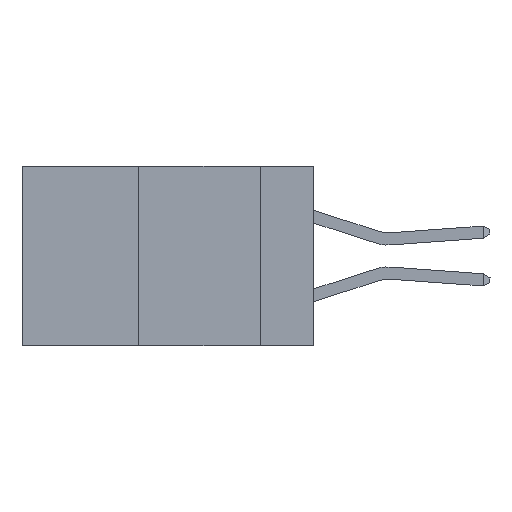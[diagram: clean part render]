
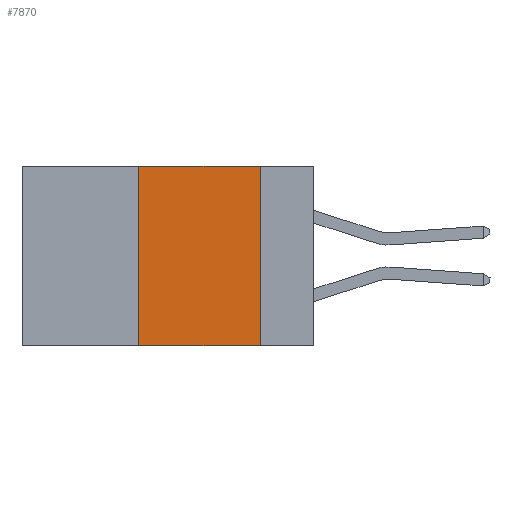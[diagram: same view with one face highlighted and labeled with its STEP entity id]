
A CAD part, left-side view. The second image highlights one B-rep face of the part: STEP entity #7870.
In plain terms, the highlighted planar face has unit normal (-1, 0, 0).
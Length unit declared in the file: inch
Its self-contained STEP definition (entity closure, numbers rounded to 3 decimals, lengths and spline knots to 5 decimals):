
#973 = ORIENTED_EDGE ( 'NONE', *, *, #4872, .F. ) ;
#1390 = FACE_OUTER_BOUND ( 'NONE', #11422, .T. ) ;
#1404 = VECTOR ( 'NONE', #12240, 39.37008 ) ;
#1565 = PLANE ( 'NONE',  #12212 ) ;
#1635 = CARTESIAN_POINT ( 'NONE',  ( 0., 0.11, -0.37 ) ) ;
#1750 = ORIENTED_EDGE ( 'NONE', *, *, #7439, .T. ) ;
#2557 = LINE ( 'NONE', #11623, #11999 ) ;
#3016 = VECTOR ( 'NONE', #4770, 39.37008 ) ;
#3152 = CARTESIAN_POINT ( 'NONE',  ( 0., 0.11, 0. ) ) ;
#3260 = VECTOR ( 'NONE', #4345, 39.37008 ) ;
#3278 = ORIENTED_EDGE ( 'NONE', *, *, #4536, .F. ) ;
#4176 = DIRECTION ( 'NONE',  ( 0., -1., 0. ) ) ;
#4233 = VERTEX_POINT ( 'NONE', #1635 ) ;
#4345 = DIRECTION ( 'NONE',  ( 0., 0., 1. ) ) ;
#4536 = EDGE_CURVE ( 'NONE', #7828, #5096, #2557, .T. ) ;
#4770 = DIRECTION ( 'NONE',  ( 0., 0., -1. ) ) ;
#4872 = EDGE_CURVE ( 'NONE', #5096, #4233, #8133, .T. ) ;
#5096 = VERTEX_POINT ( 'NONE', #3152 ) ;
#5343 = VERTEX_POINT ( 'NONE', #11072 ) ;
#5469 = DIRECTION ( 'NONE',  ( 1., 0., 0. ) ) ;
#6569 = LINE ( 'NONE', #7678, #1404 ) ;
#6802 = EDGE_CURVE ( 'NONE', #5343, #7828, #10824, .T. ) ;
#7439 = EDGE_CURVE ( 'NONE', #5343, #4233, #6569, .T. ) ;
#7678 = CARTESIAN_POINT ( 'NONE',  ( 0., 0.6, -0.37 ) ) ;
#7828 = VERTEX_POINT ( 'NONE', #11909 ) ;
#7870 = ADVANCED_FACE ( 'NONE', ( #1390 ), #1565, .F. ) ;
#8133 = LINE ( 'NONE', #11309, #3016 ) ;
#8182 = CARTESIAN_POINT ( 'NONE',  ( 0., 0.36, 0. ) ) ;
#10824 = LINE ( 'NONE', #8182, #3260 ) ;
#11072 = CARTESIAN_POINT ( 'NONE',  ( 0., 0.36, -0.37 ) ) ;
#11092 = CARTESIAN_POINT ( 'NONE',  ( 0., 0.6, 0. ) ) ;
#11107 = ORIENTED_EDGE ( 'NONE', *, *, #6802, .F. ) ;
#11309 = CARTESIAN_POINT ( 'NONE',  ( 0., 0.11, 0. ) ) ;
#11422 = EDGE_LOOP ( 'NONE', ( #973, #3278, #11107, #1750 ) ) ;
#11623 = CARTESIAN_POINT ( 'NONE',  ( 0., 0.6, 0. ) ) ;
#11909 = CARTESIAN_POINT ( 'NONE',  ( 0., 0.36, 0. ) ) ;
#11991 = DIRECTION ( 'NONE',  ( 0., 0., -1. ) ) ;
#11999 = VECTOR ( 'NONE', #4176, 39.37008 ) ;
#12212 = AXIS2_PLACEMENT_3D ( 'NONE', #11092, #5469, #11991 ) ;
#12240 = DIRECTION ( 'NONE',  ( 0., -1., 0. ) ) ;
